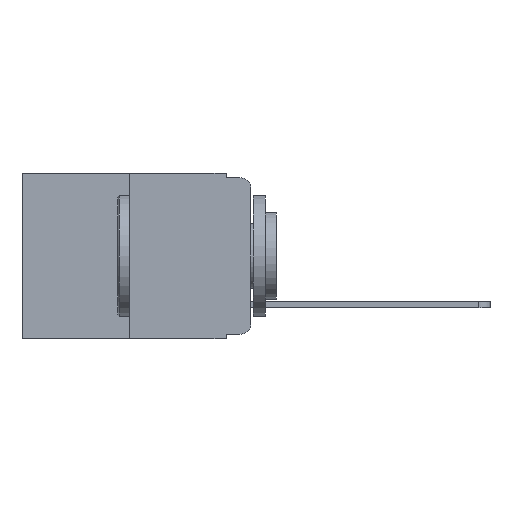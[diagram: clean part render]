
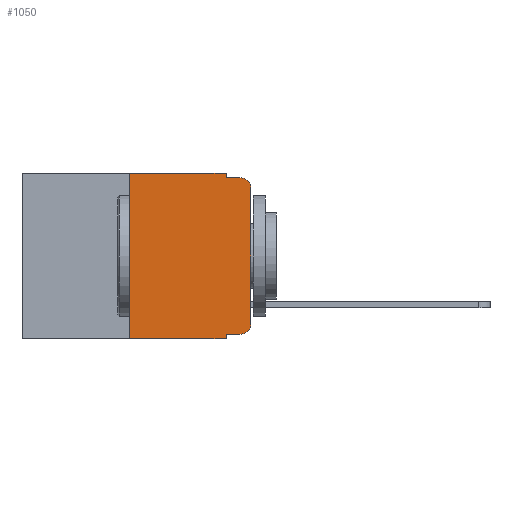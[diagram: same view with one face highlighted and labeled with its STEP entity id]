
A CAD part, left-side view. The second image highlights one B-rep face of the part: STEP entity #1050.
In plain terms, the highlighted planar face has unit normal (-1, 0, 0).
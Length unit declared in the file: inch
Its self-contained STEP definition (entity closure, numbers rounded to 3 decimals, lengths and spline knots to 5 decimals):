
#125 = DIRECTION ( 'NONE',  ( 0., 0., 1. ) ) ;
#232 = CARTESIAN_POINT ( 'NONE',  ( 0., 0.02, -0.313 ) ) ;
#946 = LINE ( 'NONE', #11618, #8906 ) ;
#1050 = ADVANCED_FACE ( 'NONE', ( #7967 ), #10404, .F. ) ;
#1098 = CARTESIAN_POINT ( 'NONE',  ( 0., 0., 0. ) ) ;
#1333 = VECTOR ( 'NONE', #9692, 39.37008 ) ;
#1355 = DIRECTION ( 'NONE',  ( 0., -1., 0. ) ) ;
#1472 = DIRECTION ( 'NONE',  ( 0., 0., -1. ) ) ;
#1806 = VERTEX_POINT ( 'NONE', #5351 ) ;
#2174 = ORIENTED_EDGE ( 'NONE', *, *, #6999, .T. ) ;
#2311 = ORIENTED_EDGE ( 'NONE', *, *, #7012, .T. ) ;
#2351 = ORIENTED_EDGE ( 'NONE', *, *, #6935, .F. ) ;
#2445 = CIRCLE ( 'NONE', #2743, 0.02 ) ;
#2523 = EDGE_LOOP ( 'NONE', ( #12720, #12812, #8397, #3083, #2940, #2918, #2622, #2351, #2311, #2174 ) ) ;
#2621 = LINE ( 'NONE', #12628, #8016 ) ;
#2622 = ORIENTED_EDGE ( 'NONE', *, *, #5788, .T. ) ;
#2743 = AXIS2_PLACEMENT_3D ( 'NONE', #10548, #4564, #11457 ) ;
#2857 = CARTESIAN_POINT ( 'NONE',  ( 0., 0., -0.313 ) ) ;
#2918 = ORIENTED_EDGE ( 'NONE', *, *, #6951, .F. ) ;
#2940 = ORIENTED_EDGE ( 'NONE', *, *, #3524, .F. ) ;
#3083 = ORIENTED_EDGE ( 'NONE', *, *, #6848, .F. ) ;
#3186 = LINE ( 'NONE', #4872, #8496 ) ;
#3470 = DIRECTION ( 'NONE',  ( 0., 0., 1. ) ) ;
#3524 = EDGE_CURVE ( 'NONE', #5920, #1806, #3186, .T. ) ;
#3992 = VERTEX_POINT ( 'NONE', #5706 ) ;
#4564 = DIRECTION ( 'NONE',  ( -1., 0., 0. ) ) ;
#4731 = VERTEX_POINT ( 'NONE', #12589 ) ;
#4872 = CARTESIAN_POINT ( 'NONE',  ( 0., 0.473, 0. ) ) ;
#5041 = VERTEX_POINT ( 'NONE', #6647 ) ;
#5052 = VECTOR ( 'NONE', #3470, 39.37008 ) ;
#5351 = CARTESIAN_POINT ( 'NONE',  ( 0., 0.051, 0. ) ) ;
#5416 = VECTOR ( 'NONE', #9364, 39.37008 ) ;
#5586 = CIRCLE ( 'NONE', #10919, 0.02 ) ;
#5706 = CARTESIAN_POINT ( 'NONE',  ( 0., 0.02, -0.333 ) ) ;
#5788 = EDGE_CURVE ( 'NONE', #5041, #7533, #7199, .T. ) ;
#5920 = VERTEX_POINT ( 'NONE', #8087 ) ;
#5927 = VECTOR ( 'NONE', #125, 39.37008 ) ;
#6286 = LINE ( 'NONE', #6946, #5927 ) ;
#6459 = AXIS2_PLACEMENT_3D ( 'NONE', #11086, #10502, #7439 ) ;
#6468 = VERTEX_POINT ( 'NONE', #2857 ) ;
#6632 = CARTESIAN_POINT ( 'NONE',  ( 0., 0.02, -0.01 ) ) ;
#6647 = CARTESIAN_POINT ( 'NONE',  ( 0., 0.25, -0.343 ) ) ;
#6793 = EDGE_CURVE ( 'NONE', #11216, #12522, #2445, .T. ) ;
#6816 = EDGE_CURVE ( 'NONE', #6468, #11216, #10356, .T. ) ;
#6848 = EDGE_CURVE ( 'NONE', #1806, #8929, #12209, .T. ) ;
#6866 = EDGE_CURVE ( 'NONE', #8929, #12522, #6936, .T. ) ;
#6935 = EDGE_CURVE ( 'NONE', #4731, #7533, #946, .T. ) ;
#6936 = LINE ( 'NONE', #12460, #1333 ) ;
#6946 = CARTESIAN_POINT ( 'NONE',  ( 0., 0.25, 0. ) ) ;
#6951 = EDGE_CURVE ( 'NONE', #5041, #5920, #6286, .T. ) ;
#6999 = EDGE_CURVE ( 'NONE', #3992, #6468, #5586, .T. ) ;
#7012 = EDGE_CURVE ( 'NONE', #4731, #3992, #2621, .T. ) ;
#7020 = DIRECTION ( 'NONE',  ( 0., -1., 0. ) ) ;
#7199 = LINE ( 'NONE', #7926, #12749 ) ;
#7439 = DIRECTION ( 'NONE',  ( 0., 0., -1. ) ) ;
#7533 = VERTEX_POINT ( 'NONE', #12167 ) ;
#7926 = CARTESIAN_POINT ( 'NONE',  ( 0., 0.473, -0.343 ) ) ;
#7967 = FACE_OUTER_BOUND ( 'NONE', #2523, .T. ) ;
#8016 = VECTOR ( 'NONE', #7020, 39.37008 ) ;
#8027 = DIRECTION ( 'NONE',  ( -1., 0., 0. ) ) ;
#8087 = CARTESIAN_POINT ( 'NONE',  ( 0., 0.25, 0. ) ) ;
#8397 = ORIENTED_EDGE ( 'NONE', *, *, #6866, .F. ) ;
#8496 = VECTOR ( 'NONE', #11729, 39.37008 ) ;
#8906 = VECTOR ( 'NONE', #12540, 39.37008 ) ;
#8929 = VERTEX_POINT ( 'NONE', #11323 ) ;
#9364 = DIRECTION ( 'NONE',  ( 0., 0., -1. ) ) ;
#9692 = DIRECTION ( 'NONE',  ( 0., -1., 0. ) ) ;
#10356 = LINE ( 'NONE', #1098, #5052 ) ;
#10404 = PLANE ( 'NONE',  #6459 ) ;
#10502 = DIRECTION ( 'NONE',  ( 1., 0., 0. ) ) ;
#10548 = CARTESIAN_POINT ( 'NONE',  ( 0., 0.02, -0.03 ) ) ;
#10764 = CARTESIAN_POINT ( 'NONE',  ( 0., 0., -0.03 ) ) ;
#10919 = AXIS2_PLACEMENT_3D ( 'NONE', #232, #8027, #1472 ) ;
#11086 = CARTESIAN_POINT ( 'NONE',  ( 0., 0.473, 0. ) ) ;
#11216 = VERTEX_POINT ( 'NONE', #10764 ) ;
#11323 = CARTESIAN_POINT ( 'NONE',  ( 0., 0.051, -0.01 ) ) ;
#11457 = DIRECTION ( 'NONE',  ( 0., 0., -1. ) ) ;
#11502 = CARTESIAN_POINT ( 'NONE',  ( 0., 0.051, 0. ) ) ;
#11618 = CARTESIAN_POINT ( 'NONE',  ( 0., 0.051, 0. ) ) ;
#11729 = DIRECTION ( 'NONE',  ( 0., -1., 0. ) ) ;
#12167 = CARTESIAN_POINT ( 'NONE',  ( 0., 0.051, -0.343 ) ) ;
#12209 = LINE ( 'NONE', #11502, #5416 ) ;
#12460 = CARTESIAN_POINT ( 'NONE',  ( 0., 0.051, -0.01 ) ) ;
#12522 = VERTEX_POINT ( 'NONE', #6632 ) ;
#12540 = DIRECTION ( 'NONE',  ( 0., 0., -1. ) ) ;
#12589 = CARTESIAN_POINT ( 'NONE',  ( 0., 0.051, -0.333 ) ) ;
#12628 = CARTESIAN_POINT ( 'NONE',  ( 0., 0.051, -0.333 ) ) ;
#12720 = ORIENTED_EDGE ( 'NONE', *, *, #6816, .T. ) ;
#12749 = VECTOR ( 'NONE', #1355, 39.37008 ) ;
#12812 = ORIENTED_EDGE ( 'NONE', *, *, #6793, .T. ) ;
